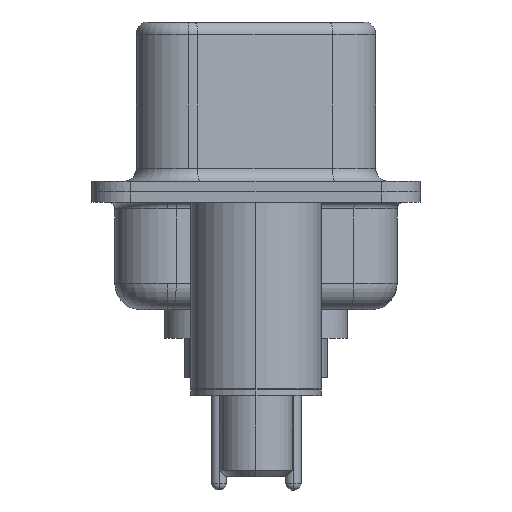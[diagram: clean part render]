
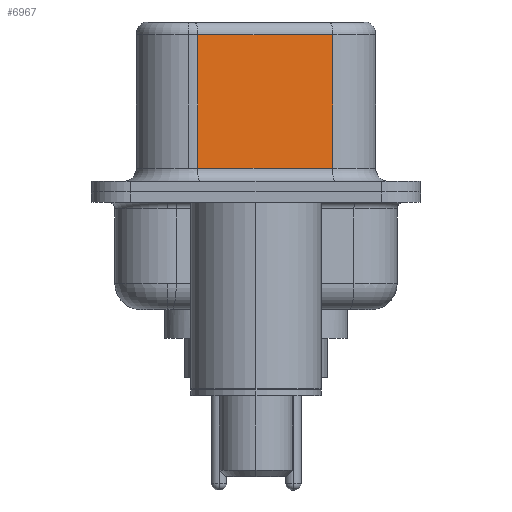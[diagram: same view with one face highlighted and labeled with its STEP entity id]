
A CAD part, left-side view. The second image highlights one B-rep face of the part: STEP entity #6967.
In plain terms, the highlighted planar face has unit normal (-0.985, -0.174, 0).
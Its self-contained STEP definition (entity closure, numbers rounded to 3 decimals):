
#823 = VECTOR ( 'NONE', #4509, 1000. ) ;
#1113 = VECTOR ( 'NONE', #19513, 1000. ) ;
#1314 = LINE ( 'NONE', #19902, #823 ) ;
#1819 = DIRECTION ( 'NONE',  ( 0., 0., -1. ) ) ;
#1933 = EDGE_CURVE ( 'NONE', #8415, #5206, #17332, .T. ) ;
#2183 = VECTOR ( 'NONE', #9605, 1000. ) ;
#2225 = VERTEX_POINT ( 'NONE', #17310 ) ;
#2240 = VERTEX_POINT ( 'NONE', #16037 ) ;
#3344 = CARTESIAN_POINT ( 'NONE',  ( 3.675, 2.233, 6.52 ) ) ;
#4509 = DIRECTION ( 'NONE',  ( -0.174, 0.985, 0. ) ) ;
#4722 = VECTOR ( 'NONE', #1819, 1000. ) ;
#5206 = VERTEX_POINT ( 'NONE', #18501 ) ;
#5908 = EDGE_CURVE ( 'NONE', #5206, #2225, #11209, .T. ) ;
#6957 = AXIS2_PLACEMENT_3D ( 'NONE', #8349, #16015, #18918 ) ;
#6967 = ADVANCED_FACE ( 'NONE', ( #18322 ), #15954, .F. ) ;
#7039 = CARTESIAN_POINT ( 'NONE',  ( 4.585, -2.927, 6.52 ) ) ;
#7066 = EDGE_CURVE ( 'NONE', #2240, #2225, #19071, .T. ) ;
#8349 = CARTESIAN_POINT ( 'NONE',  ( 4.585, -2.927, 6.52 ) ) ;
#8415 = VERTEX_POINT ( 'NONE', #13977 ) ;
#9605 = DIRECTION ( 'NONE',  ( 0.174, -0.985, 0. ) ) ;
#9875 = CARTESIAN_POINT ( 'NONE',  ( 4.585, -2.927, 0.9 ) ) ;
#10164 = EDGE_LOOP ( 'NONE', ( #20044, #10262, #18969, #18416 ) ) ;
#10262 = ORIENTED_EDGE ( 'NONE', *, *, #15442, .T. ) ;
#11209 = LINE ( 'NONE', #9875, #2183 ) ;
#13977 = CARTESIAN_POINT ( 'NONE',  ( 3.675, 2.233, 6.02 ) ) ;
#15442 = EDGE_CURVE ( 'NONE', #2240, #8415, #1314, .T. ) ;
#15954 = PLANE ( 'NONE',  #6957 ) ;
#16015 = DIRECTION ( 'NONE',  ( 0.985, 0.174, 0. ) ) ;
#16037 = CARTESIAN_POINT ( 'NONE',  ( 4.585, -2.927, 6.02 ) ) ;
#17310 = CARTESIAN_POINT ( 'NONE',  ( 4.585, -2.927, 0.9 ) ) ;
#17332 = LINE ( 'NONE', #3344, #4722 ) ;
#18322 = FACE_OUTER_BOUND ( 'NONE', #10164, .T. ) ;
#18416 = ORIENTED_EDGE ( 'NONE', *, *, #5908, .T. ) ;
#18501 = CARTESIAN_POINT ( 'NONE',  ( 3.675, 2.233, 0.9 ) ) ;
#18918 = DIRECTION ( 'NONE',  ( -0.174, 0.985, 0. ) ) ;
#18969 = ORIENTED_EDGE ( 'NONE', *, *, #1933, .T. ) ;
#19071 = LINE ( 'NONE', #7039, #1113 ) ;
#19513 = DIRECTION ( 'NONE',  ( 0., 0., -1. ) ) ;
#19902 = CARTESIAN_POINT ( 'NONE',  ( 4.585, -2.927, 6.02 ) ) ;
#20044 = ORIENTED_EDGE ( 'NONE', *, *, #7066, .F. ) ;
